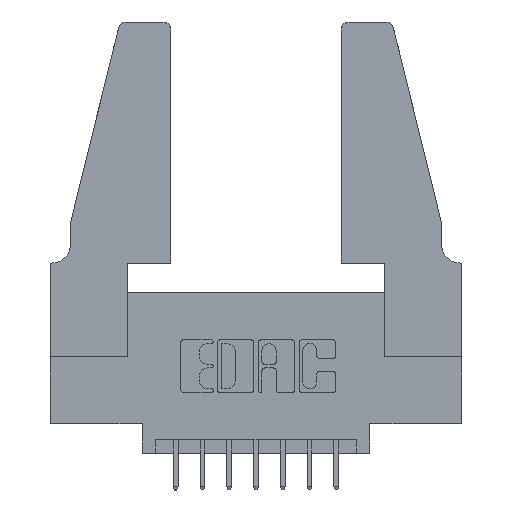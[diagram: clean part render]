
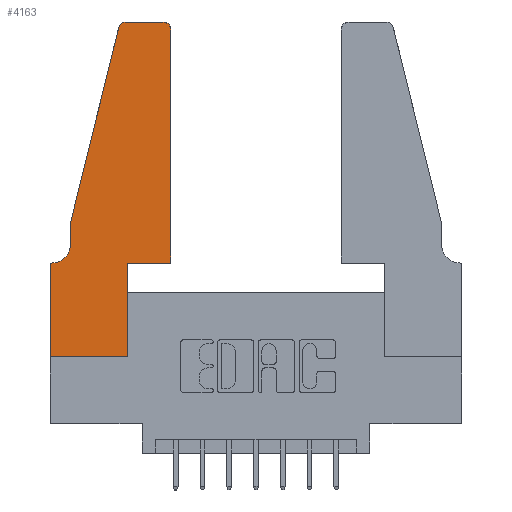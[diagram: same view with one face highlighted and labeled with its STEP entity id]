
A CAD part, top view. The second image highlights one B-rep face of the part: STEP entity #4163.
In plain terms, the highlighted planar face has unit normal (0, 0, 1).
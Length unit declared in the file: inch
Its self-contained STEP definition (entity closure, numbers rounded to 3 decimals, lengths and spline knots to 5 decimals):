
#273 = DIRECTION ( 'NONE',  ( 0., -1., 0. ) ) ;
#362 = LINE ( 'NONE', #7924, #7107 ) ;
#413 = ORIENTED_EDGE ( 'NONE', *, *, #12415, .T. ) ;
#449 = VECTOR ( 'NONE', #12460, 39.37008 ) ;
#505 = LINE ( 'NONE', #2123, #3888 ) ;
#780 = LINE ( 'NONE', #11416, #449 ) ;
#835 = CARTESIAN_POINT ( 'NONE',  ( 0.284, 1.25, 0.37 ) ) ;
#1248 = CARTESIAN_POINT ( 'NONE',  ( 0.2605, 1.25, 0.37 ) ) ;
#1704 = VECTOR ( 'NONE', #7179, 39.37008 ) ;
#1870 = ORIENTED_EDGE ( 'NONE', *, *, #7302, .T. ) ;
#2037 = VECTOR ( 'NONE', #9908, 39.37008 ) ;
#2055 = EDGE_CURVE ( 'NONE', #2395, #5532, #12131, .T. ) ;
#2123 = CARTESIAN_POINT ( 'NONE',  ( 0.0755, 0.35, 0.37 ) ) ;
#2395 = VERTEX_POINT ( 'NONE', #4094 ) ;
#2570 = EDGE_CURVE ( 'NONE', #7553, #7855, #7526, .T. ) ;
#2727 = EDGE_CURVE ( 'NONE', #9803, #3688, #2746, .T. ) ;
#2741 = AXIS2_PLACEMENT_3D ( 'NONE', #11478, #6600, #3936 ) ;
#2746 = CIRCLE ( 'NONE', #2741, 0.03 ) ;
#2808 = EDGE_CURVE ( 'NONE', #5528, #8708, #3614, .T. ) ;
#2821 = CARTESIAN_POINT ( 'NONE',  ( 0.0755, 0.5, 0.37 ) ) ;
#3375 = ORIENTED_EDGE ( 'NONE', *, *, #2570, .T. ) ;
#3416 = CARTESIAN_POINT ( 'NONE',  ( 0.25487, 1.22718, 0.37 ) ) ;
#3424 = CARTESIAN_POINT ( 'NONE',  ( 0.4505, 0.35, 0.37 ) ) ;
#3614 = CIRCLE ( 'NONE', #3810, 0.03 ) ;
#3659 = ORIENTED_EDGE ( 'NONE', *, *, #8842, .T. ) ;
#3688 = VERTEX_POINT ( 'NONE', #3416 ) ;
#3810 = AXIS2_PLACEMENT_3D ( 'NONE', #5077, #7968, #12055 ) ;
#3888 = VECTOR ( 'NONE', #12024, 39.37008 ) ;
#3922 = EDGE_LOOP ( 'NONE', ( #7683, #8331, #413, #3659, #4945, #11851, #10970, #11267, #11652, #3375, #1870, #9587 ) ) ;
#3936 = DIRECTION ( 'NONE',  ( 1., 0., 0. ) ) ;
#4065 = CARTESIAN_POINT ( 'NONE',  ( 0.2865, 0., 0.37 ) ) ;
#4094 = CARTESIAN_POINT ( 'NONE',  ( 0.0755, 0.42, 0.37 ) ) ;
#4130 = DIRECTION ( 'NONE',  ( 1., 0., 0. ) ) ;
#4163 = ADVANCED_FACE ( 'NONE', ( #9488 ), #6437, .T. ) ;
#4607 = DIRECTION ( 'NONE',  ( 0., 0., 1. ) ) ;
#4822 = LINE ( 'NONE', #9772, #10033 ) ;
#4945 = ORIENTED_EDGE ( 'NONE', *, *, #2055, .T. ) ;
#5077 = CARTESIAN_POINT ( 'NONE',  ( 0.4205, 1.22, 0.37 ) ) ;
#5122 = DIRECTION ( 'NONE',  ( -1., 0., 0. ) ) ;
#5499 = EDGE_CURVE ( 'NONE', #9621, #7553, #780, .T. ) ;
#5528 = VERTEX_POINT ( 'NONE', #5718 ) ;
#5532 = VERTEX_POINT ( 'NONE', #9465 ) ;
#5584 = VECTOR ( 'NONE', #273, 39.37008 ) ;
#5718 = CARTESIAN_POINT ( 'NONE',  ( 0.4505, 1.22, 0.37 ) ) ;
#5885 = CARTESIAN_POINT ( 'NONE',  ( 0.0755, 0.5, 0.37 ) ) ;
#6187 = EDGE_CURVE ( 'NONE', #10900, #9621, #362, .T. ) ;
#6437 = PLANE ( 'NONE',  #9781 ) ;
#6549 = CARTESIAN_POINT ( 'NONE',  ( 0.4505, 0.35, 0.37 ) ) ;
#6593 = VERTEX_POINT ( 'NONE', #2821 ) ;
#6600 = DIRECTION ( 'NONE',  ( 0., 0., 1. ) ) ;
#6716 = CARTESIAN_POINT ( 'NONE',  ( 0.4505, 0.35, 0.37 ) ) ;
#6725 = EDGE_CURVE ( 'NONE', #8708, #9803, #10006, .T. ) ;
#6778 = CARTESIAN_POINT ( 'NONE',  ( 0.0055, 0.42, 0.37 ) ) ;
#7107 = VECTOR ( 'NONE', #4130, 39.37008 ) ;
#7179 = DIRECTION ( 'NONE',  ( -0.239, -0.971, 0. ) ) ;
#7302 = EDGE_CURVE ( 'NONE', #7855, #5528, #11930, .T. ) ;
#7369 = CARTESIAN_POINT ( 'NONE',  ( 0.2865, 0.35, 0.37 ) ) ;
#7526 = LINE ( 'NONE', #6549, #9976 ) ;
#7553 = VERTEX_POINT ( 'NONE', #7369 ) ;
#7683 = ORIENTED_EDGE ( 'NONE', *, *, #6725, .T. ) ;
#7766 = DIRECTION ( 'NONE',  ( 0., 0., -1. ) ) ;
#7769 = DIRECTION ( 'NONE',  ( 0., -1., 0. ) ) ;
#7855 = VERTEX_POINT ( 'NONE', #3424 ) ;
#7924 = CARTESIAN_POINT ( 'NONE',  ( 0., 0., 0.37 ) ) ;
#7968 = DIRECTION ( 'NONE',  ( 0., 0., 1. ) ) ;
#8021 = CARTESIAN_POINT ( 'NONE',  ( 0., 0., 0.37 ) ) ;
#8131 = EDGE_CURVE ( 'NONE', #5532, #11581, #505, .T. ) ;
#8331 = ORIENTED_EDGE ( 'NONE', *, *, #2727, .T. ) ;
#8708 = VERTEX_POINT ( 'NONE', #10841 ) ;
#8842 = EDGE_CURVE ( 'NONE', #6593, #2395, #4822, .T. ) ;
#8991 = LINE ( 'NONE', #8021, #5584 ) ;
#9465 = CARTESIAN_POINT ( 'NONE',  ( 0.0055, 0.35, 0.37 ) ) ;
#9488 = FACE_OUTER_BOUND ( 'NONE', #3922, .T. ) ;
#9587 = ORIENTED_EDGE ( 'NONE', *, *, #2808, .T. ) ;
#9621 = VERTEX_POINT ( 'NONE', #4065 ) ;
#9771 = DIRECTION ( 'NONE',  ( -1., 0., 0. ) ) ;
#9772 = CARTESIAN_POINT ( 'NONE',  ( 0.0755, 0.5, 0.37 ) ) ;
#9781 = AXIS2_PLACEMENT_3D ( 'NONE', #10506, #4607, #11493 ) ;
#9803 = VERTEX_POINT ( 'NONE', #835 ) ;
#9908 = DIRECTION ( 'NONE',  ( 0., 1., 0. ) ) ;
#9976 = VECTOR ( 'NONE', #11431, 39.37008 ) ;
#10006 = LINE ( 'NONE', #1248, #11409 ) ;
#10033 = VECTOR ( 'NONE', #7769, 39.37008 ) ;
#10101 = CARTESIAN_POINT ( 'NONE',  ( 0., 0.35, 0.37 ) ) ;
#10506 = CARTESIAN_POINT ( 'NONE',  ( 0., 0.35, 0.37 ) ) ;
#10513 = CARTESIAN_POINT ( 'NONE',  ( 0., 0., 0.37 ) ) ;
#10841 = CARTESIAN_POINT ( 'NONE',  ( 0.4205, 1.25, 0.37 ) ) ;
#10900 = VERTEX_POINT ( 'NONE', #10513 ) ;
#10970 = ORIENTED_EDGE ( 'NONE', *, *, #11906, .T. ) ;
#11022 = LINE ( 'NONE', #5885, #1704 ) ;
#11267 = ORIENTED_EDGE ( 'NONE', *, *, #6187, .T. ) ;
#11409 = VECTOR ( 'NONE', #5122, 39.37008 ) ;
#11416 = CARTESIAN_POINT ( 'NONE',  ( 0.2865, 0.35, 0.37 ) ) ;
#11431 = DIRECTION ( 'NONE',  ( 1., 0., 0. ) ) ;
#11478 = CARTESIAN_POINT ( 'NONE',  ( 0.284, 1.22, 0.37 ) ) ;
#11493 = DIRECTION ( 'NONE',  ( 1., 0., 0. ) ) ;
#11581 = VERTEX_POINT ( 'NONE', #10101 ) ;
#11652 = ORIENTED_EDGE ( 'NONE', *, *, #5499, .T. ) ;
#11851 = ORIENTED_EDGE ( 'NONE', *, *, #8131, .T. ) ;
#11906 = EDGE_CURVE ( 'NONE', #11581, #10900, #8991, .T. ) ;
#11930 = LINE ( 'NONE', #6716, #2037 ) ;
#12024 = DIRECTION ( 'NONE',  ( -1., 0., 0. ) ) ;
#12055 = DIRECTION ( 'NONE',  ( 1., 0., 0. ) ) ;
#12131 = CIRCLE ( 'NONE', #12185, 0.07 ) ;
#12185 = AXIS2_PLACEMENT_3D ( 'NONE', #6778, #7766, #9771 ) ;
#12415 = EDGE_CURVE ( 'NONE', #3688, #6593, #11022, .T. ) ;
#12460 = DIRECTION ( 'NONE',  ( 0., 1., 0. ) ) ;
